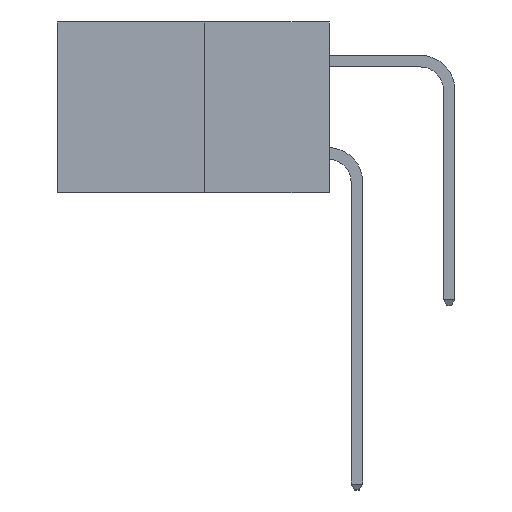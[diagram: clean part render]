
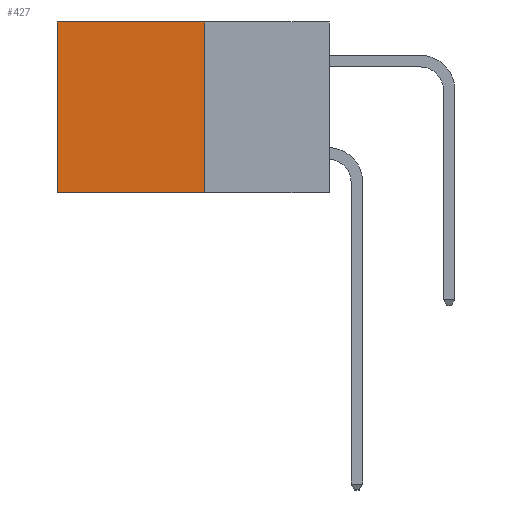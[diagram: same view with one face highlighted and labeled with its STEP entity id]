
A CAD part, left-side view. The second image highlights one B-rep face of the part: STEP entity #427.
In plain terms, the highlighted planar face has unit normal (-1, 0, 0).
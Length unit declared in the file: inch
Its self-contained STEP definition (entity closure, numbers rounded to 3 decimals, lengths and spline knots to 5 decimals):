
#22 = VERTEX_POINT ( 'NONE', #6553 ) ;
#103 = DIRECTION ( 'NONE',  ( 0., 1., 0. ) ) ;
#362 = EDGE_CURVE ( 'NONE', #6879, #1459, #1825, .T. ) ;
#427 = ADVANCED_FACE ( 'NONE', ( #5454 ), #5279, .F. ) ;
#1417 = VECTOR ( 'NONE', #8847, 39.37008 ) ;
#1459 = VERTEX_POINT ( 'NONE', #10176 ) ;
#1701 = CARTESIAN_POINT ( 'NONE',  ( 0.277, 0.27, 0. ) ) ;
#1825 = LINE ( 'NONE', #2855, #9906 ) ;
#2204 = EDGE_CURVE ( 'NONE', #6604, #22, #7938, .T. ) ;
#2206 = DIRECTION ( 'NONE',  ( 0., 0., -1. ) ) ;
#2225 = CARTESIAN_POINT ( 'NONE',  ( 0.277, 0.27, -0.37 ) ) ;
#2587 = VECTOR ( 'NONE', #2206, 39.37008 ) ;
#2855 = CARTESIAN_POINT ( 'NONE',  ( 0.277, 0.27, -0.37 ) ) ;
#2936 = DIRECTION ( 'NONE',  ( 0., 0., -1. ) ) ;
#2979 = EDGE_CURVE ( 'NONE', #22, #1459, #7316, .T. ) ;
#3703 = EDGE_LOOP ( 'NONE', ( #4240, #4247, #4260, #4261 ) ) ;
#4240 = ORIENTED_EDGE ( 'NONE', *, *, #2979, .T. ) ;
#4247 = ORIENTED_EDGE ( 'NONE', *, *, #362, .F. ) ;
#4260 = ORIENTED_EDGE ( 'NONE', *, *, #6492, .F. ) ;
#4261 = ORIENTED_EDGE ( 'NONE', *, *, #2204, .T. ) ;
#4748 = DIRECTION ( 'NONE',  ( 0., 0., -1. ) ) ;
#4822 = LINE ( 'NONE', #2225, #2587 ) ;
#5279 = PLANE ( 'NONE',  #5927 ) ;
#5454 = FACE_OUTER_BOUND ( 'NONE', #3703, .T. ) ;
#5927 = AXIS2_PLACEMENT_3D ( 'NONE', #7157, #8046, #2936 ) ;
#6492 = EDGE_CURVE ( 'NONE', #6604, #6879, #4822, .T. ) ;
#6553 = CARTESIAN_POINT ( 'NONE',  ( 0.277, 0.59, 0. ) ) ;
#6604 = VERTEX_POINT ( 'NONE', #1701 ) ;
#6879 = VERTEX_POINT ( 'NONE', #8211 ) ;
#7157 = CARTESIAN_POINT ( 'NONE',  ( 0.277, 0.27, -0.37 ) ) ;
#7265 = CARTESIAN_POINT ( 'NONE',  ( 0.277, 0.59, -0.37 ) ) ;
#7316 = LINE ( 'NONE', #7265, #7564 ) ;
#7564 = VECTOR ( 'NONE', #4748, 39.37008 ) ;
#7706 = CARTESIAN_POINT ( 'NONE',  ( 0.277, 0.27, 0. ) ) ;
#7938 = LINE ( 'NONE', #7706, #1417 ) ;
#8046 = DIRECTION ( 'NONE',  ( 1., 0., 0. ) ) ;
#8211 = CARTESIAN_POINT ( 'NONE',  ( 0.277, 0.27, -0.37 ) ) ;
#8847 = DIRECTION ( 'NONE',  ( 0., 1., 0. ) ) ;
#9906 = VECTOR ( 'NONE', #103, 39.37008 ) ;
#10176 = CARTESIAN_POINT ( 'NONE',  ( 0.277, 0.59, -0.37 ) ) ;
